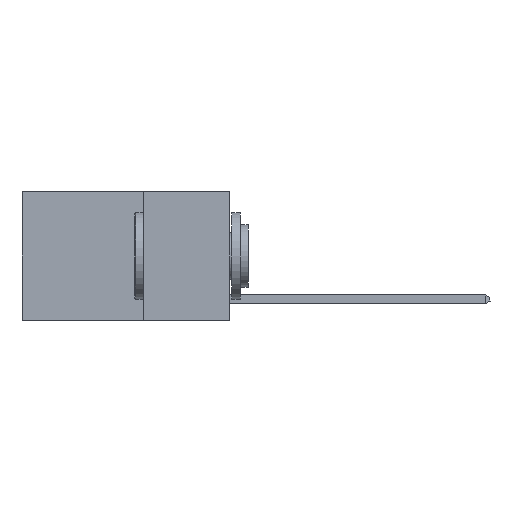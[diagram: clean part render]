
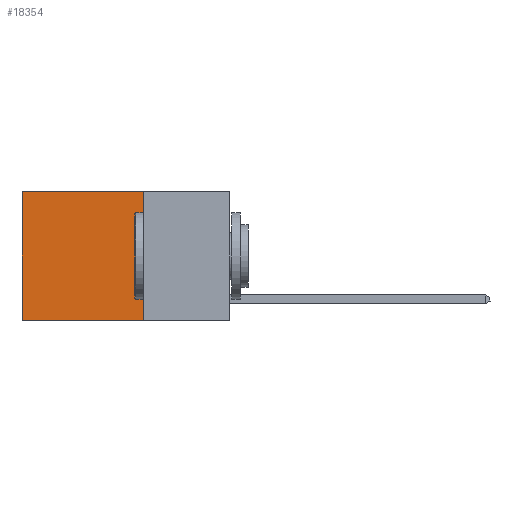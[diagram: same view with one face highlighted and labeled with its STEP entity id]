
A CAD part, left-side view. The second image highlights one B-rep face of the part: STEP entity #18354.
In plain terms, the highlighted planar face has unit normal (-1, 0, 0).
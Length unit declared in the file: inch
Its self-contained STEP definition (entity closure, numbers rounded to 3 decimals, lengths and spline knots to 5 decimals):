
#212 = VECTOR ( 'NONE', #3654, 39.37008 ) ;
#403 = VERTEX_POINT ( 'NONE', #11019 ) ;
#446 = ORIENTED_EDGE ( 'NONE', *, *, #4561, .F. ) ;
#471 = CARTESIAN_POINT ( 'NONE',  ( 0.2625, 0.25, -0.37 ) ) ;
#1220 = DIRECTION ( 'NONE',  ( 0., 1., 0. ) ) ;
#2068 = ORIENTED_EDGE ( 'NONE', *, *, #19222, .T. ) ;
#2299 = CARTESIAN_POINT ( 'NONE',  ( 0.2625, 0.25, 0. ) ) ;
#2668 = PLANE ( 'NONE',  #12134 ) ;
#3199 = FACE_OUTER_BOUND ( 'NONE', #17570, .T. ) ;
#3654 = DIRECTION ( 'NONE',  ( 0., 0., -1. ) ) ;
#4386 = LINE ( 'NONE', #13125, #212 ) ;
#4561 = EDGE_CURVE ( 'NONE', #14009, #403, #4386, .T. ) ;
#5209 = EDGE_CURVE ( 'NONE', #403, #17676, #5605, .T. ) ;
#5240 = CARTESIAN_POINT ( 'NONE',  ( 0.2625, 0.6, 0. ) ) ;
#5601 = ORIENTED_EDGE ( 'NONE', *, *, #7317, .T. ) ;
#5605 = LINE ( 'NONE', #471, #9304 ) ;
#5756 = DIRECTION ( 'NONE',  ( 1., 0., 0. ) ) ;
#6851 = DIRECTION ( 'NONE',  ( 0., 0., -1. ) ) ;
#7317 = EDGE_CURVE ( 'NONE', #14009, #9752, #10597, .T. ) ;
#7823 = VECTOR ( 'NONE', #6851, 39.37008 ) ;
#8070 = LINE ( 'NONE', #5240, #7823 ) ;
#9304 = VECTOR ( 'NONE', #11541, 39.37008 ) ;
#9583 = ORIENTED_EDGE ( 'NONE', *, *, #5209, .F. ) ;
#9752 = VERTEX_POINT ( 'NONE', #19278 ) ;
#10597 = LINE ( 'NONE', #18529, #10792 ) ;
#10792 = VECTOR ( 'NONE', #1220, 39.37008 ) ;
#11019 = CARTESIAN_POINT ( 'NONE',  ( 0.2625, 0.25, -0.37 ) ) ;
#11541 = DIRECTION ( 'NONE',  ( 0., 1., 0. ) ) ;
#12134 = AXIS2_PLACEMENT_3D ( 'NONE', #18351, #5756, #19861 ) ;
#13125 = CARTESIAN_POINT ( 'NONE',  ( 0.2625, 0.25, 0. ) ) ;
#14009 = VERTEX_POINT ( 'NONE', #2299 ) ;
#16239 = CARTESIAN_POINT ( 'NONE',  ( 0.2625, 0.6, -0.37 ) ) ;
#17570 = EDGE_LOOP ( 'NONE', ( #2068, #9583, #446, #5601 ) ) ;
#17676 = VERTEX_POINT ( 'NONE', #16239 ) ;
#18351 = CARTESIAN_POINT ( 'NONE',  ( 0.2625, 0.25, 0. ) ) ;
#18354 = ADVANCED_FACE ( 'NONE', ( #3199 ), #2668, .F. ) ;
#18529 = CARTESIAN_POINT ( 'NONE',  ( 0.2625, 0.25, 0. ) ) ;
#19222 = EDGE_CURVE ( 'NONE', #9752, #17676, #8070, .T. ) ;
#19278 = CARTESIAN_POINT ( 'NONE',  ( 0.2625, 0.6, 0. ) ) ;
#19861 = DIRECTION ( 'NONE',  ( 0., 0., -1. ) ) ;
